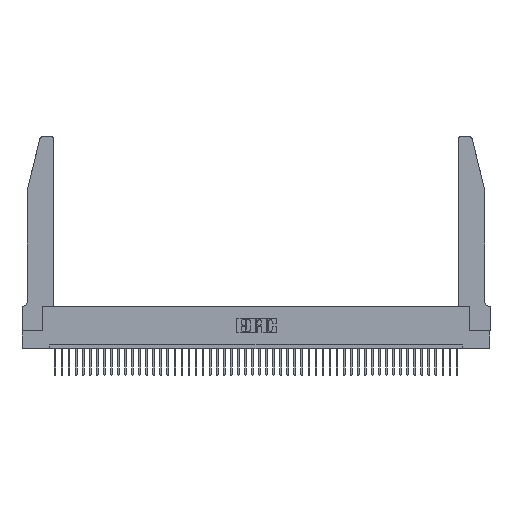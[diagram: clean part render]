
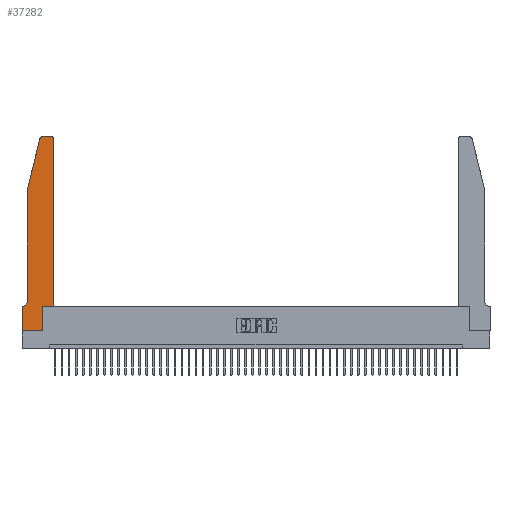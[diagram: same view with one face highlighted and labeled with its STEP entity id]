
A CAD part, top view. The second image highlights one B-rep face of the part: STEP entity #37282.
In plain terms, the highlighted planar face has unit normal (0, 0, 1).
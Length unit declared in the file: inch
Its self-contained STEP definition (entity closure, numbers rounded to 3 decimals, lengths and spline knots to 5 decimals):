
#167 = DIRECTION ( 'NONE',  ( 1., 0., 0. ) ) ;
#235 = EDGE_CURVE ( 'NONE', #15026, #4139, #18654, .T. ) ;
#547 = VECTOR ( 'NONE', #40877, 39.37008 ) ;
#822 = EDGE_CURVE ( 'NONE', #36474, #7513, #28060, .T. ) ;
#1003 = LINE ( 'NONE', #14300, #2758 ) ;
#1169 = ORIENTED_EDGE ( 'NONE', *, *, #235, .T. ) ;
#1250 = EDGE_CURVE ( 'NONE', #9037, #14512, #34135, .T. ) ;
#1478 = CARTESIAN_POINT ( 'NONE',  ( 0.284, 2.72, 0.37 ) ) ;
#1762 = CARTESIAN_POINT ( 'NONE',  ( 0.0755, 0.42, 0.37 ) ) ;
#2039 = EDGE_CURVE ( 'NONE', #36367, #14286, #11145, .T. ) ;
#2059 = ORIENTED_EDGE ( 'NONE', *, *, #27668, .T. ) ;
#2111 = EDGE_CURVE ( 'NONE', #7513, #27556, #16258, .T. ) ;
#2699 = CARTESIAN_POINT ( 'NONE',  ( 0., 0.35, 0.37 ) ) ;
#2733 = DIRECTION ( 'NONE',  ( 0., 1., 0. ) ) ;
#2758 = VECTOR ( 'NONE', #2733, 39.37008 ) ;
#2889 = ORIENTED_EDGE ( 'NONE', *, *, #822, .T. ) ;
#3021 = ORIENTED_EDGE ( 'NONE', *, *, #2039, .T. ) ;
#3220 = EDGE_CURVE ( 'NONE', #8337, #36474, #1003, .T. ) ;
#3563 = CIRCLE ( 'NONE', #9497, 0.03 ) ;
#4139 = VERTEX_POINT ( 'NONE', #32205 ) ;
#4211 = CARTESIAN_POINT ( 'NONE',  ( 0.0755, 2., 0.37 ) ) ;
#4450 = ORIENTED_EDGE ( 'NONE', *, *, #38198, .T. ) ;
#5221 = ORIENTED_EDGE ( 'NONE', *, *, #25920, .T. ) ;
#5615 = DIRECTION ( 'NONE',  ( 0., 0., -1. ) ) ;
#5619 = CARTESIAN_POINT ( 'NONE',  ( 0.2605, 2.75, 0.37 ) ) ;
#5655 = VECTOR ( 'NONE', #167, 39.37008 ) ;
#6888 = CARTESIAN_POINT ( 'NONE',  ( 0.4505, 0.35, 0.37 ) ) ;
#7513 = VERTEX_POINT ( 'NONE', #6888 ) ;
#7767 = VECTOR ( 'NONE', #40060, 39.37008 ) ;
#8337 = VERTEX_POINT ( 'NONE', #12026 ) ;
#8419 = CARTESIAN_POINT ( 'NONE',  ( 0.0055, 0.42, 0.37 ) ) ;
#8937 = LINE ( 'NONE', #44269, #39145 ) ;
#8975 = ORIENTED_EDGE ( 'NONE', *, *, #11038, .T. ) ;
#9037 = VERTEX_POINT ( 'NONE', #1762 ) ;
#9497 = AXIS2_PLACEMENT_3D ( 'NONE', #31797, #45916, #39593 ) ;
#9605 = FACE_OUTER_BOUND ( 'NONE', #42850, .T. ) ;
#10212 = CARTESIAN_POINT ( 'NONE',  ( 0.0755, 2., 0.37 ) ) ;
#10328 = VECTOR ( 'NONE', #41902, 39.37008 ) ;
#11038 = EDGE_CURVE ( 'NONE', #17774, #14173, #8937, .T. ) ;
#11145 = LINE ( 'NONE', #5619, #547 ) ;
#11361 = DIRECTION ( 'NONE',  ( -0.239, -0.971, 0. ) ) ;
#12026 = CARTESIAN_POINT ( 'NONE',  ( 0.2865, 0., 0.37 ) ) ;
#13554 = CARTESIAN_POINT ( 'NONE',  ( 0., 0.35, 0.37 ) ) ;
#14173 = VERTEX_POINT ( 'NONE', #10212 ) ;
#14286 = VERTEX_POINT ( 'NONE', #17338 ) ;
#14300 = CARTESIAN_POINT ( 'NONE',  ( 0.2865, 0.35, 0.37 ) ) ;
#14357 = AXIS2_PLACEMENT_3D ( 'NONE', #1478, #16358, #26475 ) ;
#14512 = VERTEX_POINT ( 'NONE', #21682 ) ;
#14554 = DIRECTION ( 'NONE',  ( 0., -1., 0. ) ) ;
#15026 = VERTEX_POINT ( 'NONE', #2699 ) ;
#15048 = DIRECTION ( 'NONE',  ( -1., 0., 0. ) ) ;
#15186 = EDGE_CURVE ( 'NONE', #4139, #8337, #41497, .T. ) ;
#16258 = LINE ( 'NONE', #25687, #7767 ) ;
#16358 = DIRECTION ( 'NONE',  ( 0., 0., 1. ) ) ;
#17176 = DIRECTION ( 'NONE',  ( 0., 0., 1. ) ) ;
#17338 = CARTESIAN_POINT ( 'NONE',  ( 0.284, 2.75, 0.37 ) ) ;
#17519 = AXIS2_PLACEMENT_3D ( 'NONE', #13554, #17176, #28083 ) ;
#17774 = VERTEX_POINT ( 'NONE', #42056 ) ;
#17900 = ORIENTED_EDGE ( 'NONE', *, *, #15186, .T. ) ;
#18374 = ORIENTED_EDGE ( 'NONE', *, *, #41721, .T. ) ;
#18654 = LINE ( 'NONE', #40163, #28740 ) ;
#21682 = CARTESIAN_POINT ( 'NONE',  ( 0.0055, 0.35, 0.37 ) ) ;
#21812 = LINE ( 'NONE', #4211, #32437 ) ;
#22669 = DIRECTION ( 'NONE',  ( 1., 0., 0. ) ) ;
#22932 = CIRCLE ( 'NONE', #14357, 0.03 ) ;
#23488 = ORIENTED_EDGE ( 'NONE', *, *, #2111, .T. ) ;
#25687 = CARTESIAN_POINT ( 'NONE',  ( 0.4505, 0.35, 0.37 ) ) ;
#25920 = EDGE_CURVE ( 'NONE', #27556, #36367, #3563, .T. ) ;
#26475 = DIRECTION ( 'NONE',  ( 1., 0., 0. ) ) ;
#27556 = VERTEX_POINT ( 'NONE', #31028 ) ;
#27668 = EDGE_CURVE ( 'NONE', #14286, #17774, #22932, .T. ) ;
#27814 = AXIS2_PLACEMENT_3D ( 'NONE', #8419, #5615, #15048 ) ;
#28060 = LINE ( 'NONE', #39820, #5655 ) ;
#28083 = DIRECTION ( 'NONE',  ( 1., 0., 0. ) ) ;
#28740 = VECTOR ( 'NONE', #36553, 39.37008 ) ;
#30809 = VECTOR ( 'NONE', #22669, 39.37008 ) ;
#31028 = CARTESIAN_POINT ( 'NONE',  ( 0.4505, 2.72, 0.37 ) ) ;
#31639 = PLANE ( 'NONE',  #17519 ) ;
#31797 = CARTESIAN_POINT ( 'NONE',  ( 0.4205, 2.72, 0.37 ) ) ;
#32205 = CARTESIAN_POINT ( 'NONE',  ( 0., 0., 0.37 ) ) ;
#32437 = VECTOR ( 'NONE', #14554, 39.37008 ) ;
#34135 = CIRCLE ( 'NONE', #27814, 0.07 ) ;
#35134 = CARTESIAN_POINT ( 'NONE',  ( 0.0755, 0.35, 0.37 ) ) ;
#36367 = VERTEX_POINT ( 'NONE', #44211 ) ;
#36474 = VERTEX_POINT ( 'NONE', #44703 ) ;
#36553 = DIRECTION ( 'NONE',  ( 0., -1., 0. ) ) ;
#36607 = LINE ( 'NONE', #35134, #10328 ) ;
#36871 = ORIENTED_EDGE ( 'NONE', *, *, #3220, .T. ) ;
#37205 = CARTESIAN_POINT ( 'NONE',  ( 0., 0., 0.37 ) ) ;
#37282 = ADVANCED_FACE ( 'NONE', ( #9605 ), #31639, .T. ) ;
#38198 = EDGE_CURVE ( 'NONE', #14173, #9037, #21812, .T. ) ;
#39145 = VECTOR ( 'NONE', #11361, 39.37008 ) ;
#39593 = DIRECTION ( 'NONE',  ( 1., 0., 0. ) ) ;
#39820 = CARTESIAN_POINT ( 'NONE',  ( 0.4505, 0.35, 0.37 ) ) ;
#40060 = DIRECTION ( 'NONE',  ( 0., 1., 0. ) ) ;
#40163 = CARTESIAN_POINT ( 'NONE',  ( 0., 0., 0.37 ) ) ;
#40877 = DIRECTION ( 'NONE',  ( -1., 0., 0. ) ) ;
#41497 = LINE ( 'NONE', #37205, #30809 ) ;
#41721 = EDGE_CURVE ( 'NONE', #14512, #15026, #36607, .T. ) ;
#41902 = DIRECTION ( 'NONE',  ( -1., 0., 0. ) ) ;
#42056 = CARTESIAN_POINT ( 'NONE',  ( 0.25487, 2.72718, 0.37 ) ) ;
#42844 = ORIENTED_EDGE ( 'NONE', *, *, #1250, .T. ) ;
#42850 = EDGE_LOOP ( 'NONE', ( #3021, #2059, #8975, #4450, #42844, #18374, #1169, #17900, #36871, #2889, #23488, #5221 ) ) ;
#44211 = CARTESIAN_POINT ( 'NONE',  ( 0.4205, 2.75, 0.37 ) ) ;
#44269 = CARTESIAN_POINT ( 'NONE',  ( 0.0755, 2., 0.37 ) ) ;
#44703 = CARTESIAN_POINT ( 'NONE',  ( 0.2865, 0.35, 0.37 ) ) ;
#45916 = DIRECTION ( 'NONE',  ( 0., 0., 1. ) ) ;
